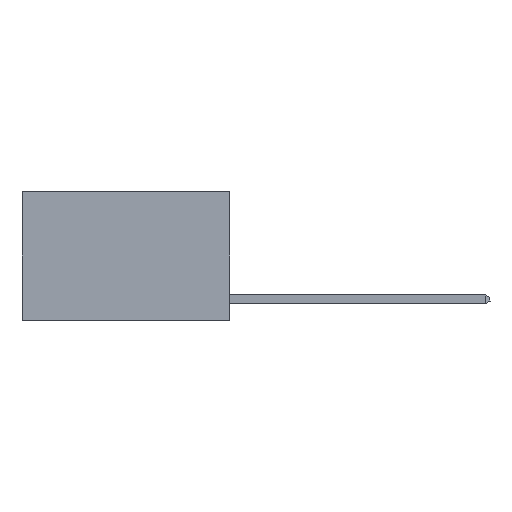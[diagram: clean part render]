
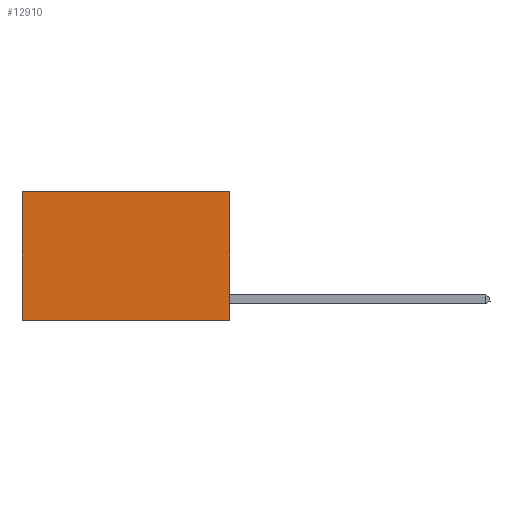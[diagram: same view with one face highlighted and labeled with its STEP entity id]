
A CAD part, left-side view. The second image highlights one B-rep face of the part: STEP entity #12910.
In plain terms, the highlighted planar face has unit normal (-1, 0, 0).
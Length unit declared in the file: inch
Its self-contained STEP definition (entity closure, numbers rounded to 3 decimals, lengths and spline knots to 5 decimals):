
#340 = LINE ( 'NONE', #10345, #21520 ) ;
#662 = CARTESIAN_POINT ( 'NONE',  ( 0.2625, 0.6, -0.37 ) ) ;
#1813 = PLANE ( 'NONE',  #14557 ) ;
#2018 = ORIENTED_EDGE ( 'NONE', *, *, #21492, .F. ) ;
#2390 = DIRECTION ( 'NONE',  ( 0., 0., -1. ) ) ;
#2637 = EDGE_LOOP ( 'NONE', ( #24010, #10050, #2018, #13799 ) ) ;
#3718 = DIRECTION ( 'NONE',  ( 1., 0., 0. ) ) ;
#4059 = EDGE_CURVE ( 'NONE', #6177, #19174, #19745, .T. ) ;
#4634 = VERTEX_POINT ( 'NONE', #18012 ) ;
#6177 = VERTEX_POINT ( 'NONE', #7252 ) ;
#6414 = CARTESIAN_POINT ( 'NONE',  ( 0.2625, 0., 0. ) ) ;
#7252 = CARTESIAN_POINT ( 'NONE',  ( 0.2625, 0.6, 0. ) ) ;
#8530 = EDGE_CURVE ( 'NONE', #16359, #6177, #10336, .T. ) ;
#9045 = FACE_OUTER_BOUND ( 'NONE', #2637, .T. ) ;
#9604 = EDGE_CURVE ( 'NONE', #4634, #19174, #10271, .T. ) ;
#9816 = CARTESIAN_POINT ( 'NONE',  ( 0.2625, 0.6, 0. ) ) ;
#10050 = ORIENTED_EDGE ( 'NONE', *, *, #9604, .F. ) ;
#10168 = DIRECTION ( 'NONE',  ( 0., 1., 0. ) ) ;
#10271 = LINE ( 'NONE', #22862, #17005 ) ;
#10336 = LINE ( 'NONE', #6414, #14745 ) ;
#10345 = CARTESIAN_POINT ( 'NONE',  ( 0.2625, 0., 0. ) ) ;
#12910 = ADVANCED_FACE ( 'NONE', ( #9045 ), #1813, .F. ) ;
#13799 = ORIENTED_EDGE ( 'NONE', *, *, #8530, .T. ) ;
#13948 = DIRECTION ( 'NONE',  ( 0., 0., -1. ) ) ;
#14557 = AXIS2_PLACEMENT_3D ( 'NONE', #22453, #3718, #2390 ) ;
#14745 = VECTOR ( 'NONE', #10168, 39.37008 ) ;
#15009 = DIRECTION ( 'NONE',  ( 0., 0., -1. ) ) ;
#15071 = VECTOR ( 'NONE', #15009, 39.37008 ) ;
#16359 = VERTEX_POINT ( 'NONE', #23612 ) ;
#17005 = VECTOR ( 'NONE', #23035, 39.37008 ) ;
#18012 = CARTESIAN_POINT ( 'NONE',  ( 0.2625, 0., -0.37 ) ) ;
#19174 = VERTEX_POINT ( 'NONE', #662 ) ;
#19745 = LINE ( 'NONE', #9816, #15071 ) ;
#21492 = EDGE_CURVE ( 'NONE', #16359, #4634, #340, .T. ) ;
#21520 = VECTOR ( 'NONE', #13948, 39.37008 ) ;
#22453 = CARTESIAN_POINT ( 'NONE',  ( 0.2625, 0., 0. ) ) ;
#22862 = CARTESIAN_POINT ( 'NONE',  ( 0.2625, 0., -0.37 ) ) ;
#23035 = DIRECTION ( 'NONE',  ( 0., 1., 0. ) ) ;
#23612 = CARTESIAN_POINT ( 'NONE',  ( 0.2625, 0., 0. ) ) ;
#24010 = ORIENTED_EDGE ( 'NONE', *, *, #4059, .T. ) ;
